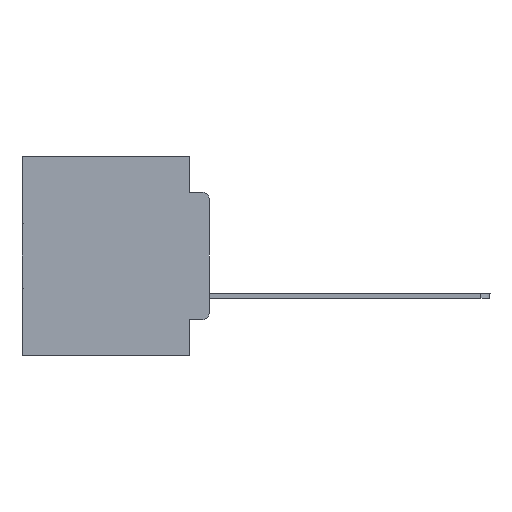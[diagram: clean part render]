
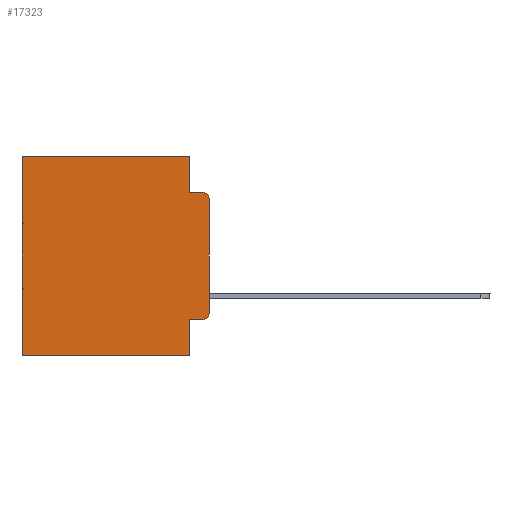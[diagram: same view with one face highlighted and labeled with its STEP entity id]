
A CAD part, left-side view. The second image highlights one B-rep face of the part: STEP entity #17323.
In plain terms, the highlighted planar face has unit normal (-1, 0, 0).
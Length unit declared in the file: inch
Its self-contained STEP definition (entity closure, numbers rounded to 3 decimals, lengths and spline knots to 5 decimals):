
#92 = PLANE ( 'NONE',  #5675 ) ;
#103 = CARTESIAN_POINT ( 'NONE',  ( 0.298, 0., -0.1085 ) ) ;
#128 = CARTESIAN_POINT ( 'NONE',  ( 0.298, 0.051, -0.4115 ) ) ;
#146 = CARTESIAN_POINT ( 'NONE',  ( 0.298, 0.02, -0.4115 ) ) ;
#554 = CARTESIAN_POINT ( 'NONE',  ( 0.298, 0., -0.3915 ) ) ;
#1143 = CARTESIAN_POINT ( 'NONE',  ( 0.298, 0.473, 0. ) ) ;
#1750 = LINE ( 'NONE', #17898, #23975 ) ;
#1853 = LINE ( 'NONE', #31131, #17509 ) ;
#1863 = ORIENTED_EDGE ( 'NONE', *, *, #16820, .T. ) ;
#2523 = LINE ( 'NONE', #128, #26883 ) ;
#3698 = EDGE_CURVE ( 'NONE', #25231, #8046, #21834, .T. ) ;
#3734 = CARTESIAN_POINT ( 'NONE',  ( 0.298, 0.02, -0.3915 ) ) ;
#3895 = DIRECTION ( 'NONE',  ( -1., 0., 0. ) ) ;
#5274 = CARTESIAN_POINT ( 'NONE',  ( 0.298, 0.051, -0.0885 ) ) ;
#5675 = AXIS2_PLACEMENT_3D ( 'NONE', #31126, #16879, #9455 ) ;
#6769 = DIRECTION ( 'NONE',  ( 0., 0., -1. ) ) ;
#6868 = EDGE_CURVE ( 'NONE', #7323, #30543, #2523, .T. ) ;
#7153 = ORIENTED_EDGE ( 'NONE', *, *, #16795, .T. ) ;
#7290 = CARTESIAN_POINT ( 'NONE',  ( 0.298, 0., -0.5 ) ) ;
#7323 = VERTEX_POINT ( 'NONE', #17646 ) ;
#7424 = ORIENTED_EDGE ( 'NONE', *, *, #12684, .T. ) ;
#8011 = VECTOR ( 'NONE', #26337, 39.37008 ) ;
#8046 = VERTEX_POINT ( 'NONE', #25967 ) ;
#8082 = CARTESIAN_POINT ( 'NONE',  ( 0.298, 0.02, -0.1085 ) ) ;
#8260 = DIRECTION ( 'NONE',  ( 0., 0., -1. ) ) ;
#9066 = VECTOR ( 'NONE', #10276, 39.37008 ) ;
#9455 = DIRECTION ( 'NONE',  ( 0., 0., -1. ) ) ;
#9493 = CARTESIAN_POINT ( 'NONE',  ( 0.298, 0.473, -0.5 ) ) ;
#9634 = VERTEX_POINT ( 'NONE', #9493 ) ;
#9802 = DIRECTION ( 'NONE',  ( 0., -1., 0. ) ) ;
#10016 = EDGE_CURVE ( 'NONE', #12023, #25231, #1853, .T. ) ;
#10276 = DIRECTION ( 'NONE',  ( 0., 1., 0. ) ) ;
#10434 = LINE ( 'NONE', #7290, #9066 ) ;
#11175 = VERTEX_POINT ( 'NONE', #103 ) ;
#11527 = ORIENTED_EDGE ( 'NONE', *, *, #10016, .F. ) ;
#11661 = EDGE_CURVE ( 'NONE', #7323, #23027, #11946, .T. ) ;
#11946 = LINE ( 'NONE', #18757, #8011 ) ;
#12023 = VERTEX_POINT ( 'NONE', #25671 ) ;
#12139 = ORIENTED_EDGE ( 'NONE', *, *, #6868, .T. ) ;
#12248 = ORIENTED_EDGE ( 'NONE', *, *, #30569, .F. ) ;
#12684 = EDGE_CURVE ( 'NONE', #12023, #18049, #26575, .T. ) ;
#13381 = DIRECTION ( 'NONE',  ( 0., 0., -1. ) ) ;
#14193 = FACE_OUTER_BOUND ( 'NONE', #22987, .T. ) ;
#14983 = CARTESIAN_POINT ( 'NONE',  ( 0.298, 0.051, -0.5 ) ) ;
#15041 = LINE ( 'NONE', #15676, #29395 ) ;
#15676 = CARTESIAN_POINT ( 'NONE',  ( 0.298, 0.473, 0. ) ) ;
#16795 = EDGE_CURVE ( 'NONE', #18049, #9634, #15041, .T. ) ;
#16820 = EDGE_CURVE ( 'NONE', #11175, #8046, #18279, .T. ) ;
#16879 = DIRECTION ( 'NONE',  ( 1., 0., 0. ) ) ;
#17323 = ADVANCED_FACE ( 'NONE', ( #14193 ), #92, .F. ) ;
#17472 = VERTEX_POINT ( 'NONE', #554 ) ;
#17509 = VECTOR ( 'NONE', #6769, 39.37008 ) ;
#17646 = CARTESIAN_POINT ( 'NONE',  ( 0.298, 0.051, -0.4115 ) ) ;
#17766 = ORIENTED_EDGE ( 'NONE', *, *, #23128, .T. ) ;
#17898 = CARTESIAN_POINT ( 'NONE',  ( 0.298, 0., 0. ) ) ;
#18049 = VERTEX_POINT ( 'NONE', #1143 ) ;
#18279 = CIRCLE ( 'NONE', #22320, 0.02 ) ;
#18757 = CARTESIAN_POINT ( 'NONE',  ( 0.298, 0.051, 0. ) ) ;
#19877 = ORIENTED_EDGE ( 'NONE', *, *, #11661, .F. ) ;
#21698 = DIRECTION ( 'NONE',  ( 0., 1., 0. ) ) ;
#21834 = LINE ( 'NONE', #24366, #25123 ) ;
#22194 = VECTOR ( 'NONE', #21698, 39.37008 ) ;
#22320 = AXIS2_PLACEMENT_3D ( 'NONE', #8082, #22791, #25314 ) ;
#22791 = DIRECTION ( 'NONE',  ( -1., 0., 0. ) ) ;
#22987 = EDGE_LOOP ( 'NONE', ( #27213, #1863, #23399, #11527, #7424, #7153, #12248, #19877, #12139, #17766 ) ) ;
#23027 = VERTEX_POINT ( 'NONE', #14983 ) ;
#23128 = EDGE_CURVE ( 'NONE', #30543, #17472, #28970, .T. ) ;
#23399 = ORIENTED_EDGE ( 'NONE', *, *, #3698, .F. ) ;
#23748 = DIRECTION ( 'NONE',  ( 0., -1., 0. ) ) ;
#23975 = VECTOR ( 'NONE', #8260, 39.37008 ) ;
#24037 = EDGE_CURVE ( 'NONE', #11175, #17472, #1750, .T. ) ;
#24366 = CARTESIAN_POINT ( 'NONE',  ( 0.298, 0.051, -0.0885 ) ) ;
#25001 = DIRECTION ( 'NONE',  ( 0., 0., -1. ) ) ;
#25123 = VECTOR ( 'NONE', #23748, 39.37008 ) ;
#25231 = VERTEX_POINT ( 'NONE', #5274 ) ;
#25314 = DIRECTION ( 'NONE',  ( 0., 0., -1. ) ) ;
#25671 = CARTESIAN_POINT ( 'NONE',  ( 0.298, 0.051, 0. ) ) ;
#25967 = CARTESIAN_POINT ( 'NONE',  ( 0.298, 0.02, -0.0885 ) ) ;
#26337 = DIRECTION ( 'NONE',  ( 0., 0., -1. ) ) ;
#26416 = CARTESIAN_POINT ( 'NONE',  ( 0.298, 0., 0. ) ) ;
#26575 = LINE ( 'NONE', #26416, #22194 ) ;
#26883 = VECTOR ( 'NONE', #9802, 39.37008 ) ;
#27213 = ORIENTED_EDGE ( 'NONE', *, *, #24037, .F. ) ;
#28970 = CIRCLE ( 'NONE', #29471, 0.02 ) ;
#29395 = VECTOR ( 'NONE', #25001, 39.37008 ) ;
#29471 = AXIS2_PLACEMENT_3D ( 'NONE', #3734, #3895, #13381 ) ;
#30543 = VERTEX_POINT ( 'NONE', #146 ) ;
#30569 = EDGE_CURVE ( 'NONE', #23027, #9634, #10434, .T. ) ;
#31126 = CARTESIAN_POINT ( 'NONE',  ( 0.298, 0., 0. ) ) ;
#31131 = CARTESIAN_POINT ( 'NONE',  ( 0.298, 0.051, 0. ) ) ;
